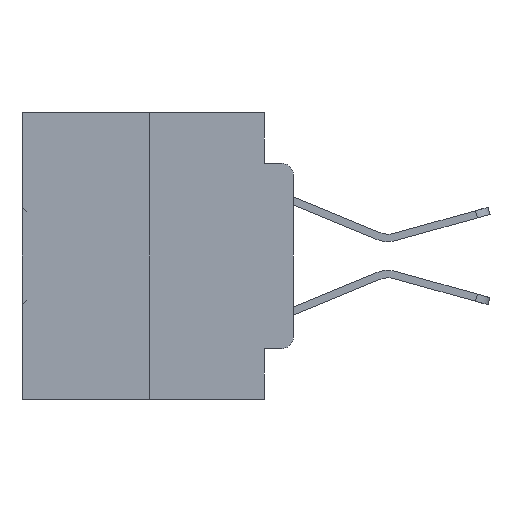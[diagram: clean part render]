
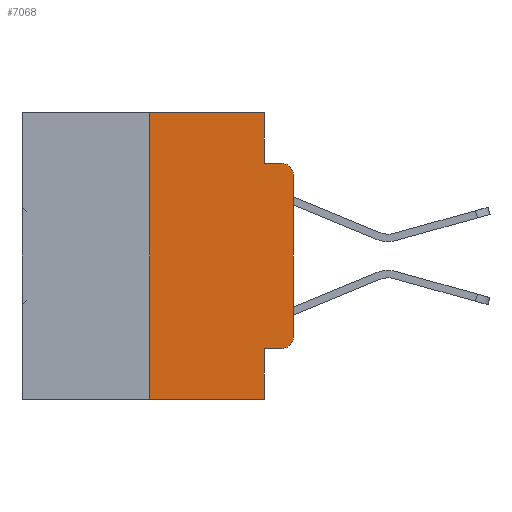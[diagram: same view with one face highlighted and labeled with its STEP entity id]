
A CAD part, left-side view. The second image highlights one B-rep face of the part: STEP entity #7068.
In plain terms, the highlighted planar face has unit normal (-1, 0, 0).
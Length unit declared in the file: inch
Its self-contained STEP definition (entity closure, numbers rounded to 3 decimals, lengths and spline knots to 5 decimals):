
#112 = AXIS2_PLACEMENT_3D ( 'NONE', #9538, #2416, #32517 ) ;
#636 = DIRECTION ( 'NONE',  ( 0., -1., 0. ) ) ;
#711 = LINE ( 'NONE', #2052, #6898 ) ;
#932 = EDGE_LOOP ( 'NONE', ( #11861, #26290, #3671, #23838, #28894, #10407, #30851, #18603, #33678, #1283 ) ) ;
#1232 = LINE ( 'NONE', #3063, #8233 ) ;
#1283 = ORIENTED_EDGE ( 'NONE', *, *, #22649, .T. ) ;
#1647 = EDGE_CURVE ( 'NONE', #32151, #18116, #25180, .T. ) ;
#2052 = CARTESIAN_POINT ( 'NONE',  ( 0., 0.051, -0.4115 ) ) ;
#2175 = CARTESIAN_POINT ( 'NONE',  ( 0., 0., -0.3915 ) ) ;
#2416 = DIRECTION ( 'NONE',  ( 1., 0., 0. ) ) ;
#2789 = CARTESIAN_POINT ( 'NONE',  ( 0., 0.25, 0. ) ) ;
#2957 = CARTESIAN_POINT ( 'NONE',  ( 0., 0., 0. ) ) ;
#3063 = CARTESIAN_POINT ( 'NONE',  ( 0., 0.473, -0.5 ) ) ;
#3671 = ORIENTED_EDGE ( 'NONE', *, *, #6938, .F. ) ;
#3848 = EDGE_CURVE ( 'NONE', #8565, #4124, #26634, .T. ) ;
#3994 = VECTOR ( 'NONE', #31921, 39.37008 ) ;
#4005 = DIRECTION ( 'NONE',  ( 0., -1., 0. ) ) ;
#4124 = VERTEX_POINT ( 'NONE', #25861 ) ;
#4366 = EDGE_CURVE ( 'NONE', #9335, #27216, #25786, .T. ) ;
#5711 = DIRECTION ( 'NONE',  ( 0., -1., 0. ) ) ;
#6165 = CARTESIAN_POINT ( 'NONE',  ( 0., 0.02, -0.3915 ) ) ;
#6453 = CARTESIAN_POINT ( 'NONE',  ( 0., 0.25, -0.5 ) ) ;
#6898 = VECTOR ( 'NONE', #25850, 39.37008 ) ;
#6938 = EDGE_CURVE ( 'NONE', #21971, #18116, #22392, .T. ) ;
#7068 = ADVANCED_FACE ( 'NONE', ( #32167 ), #7983, .F. ) ;
#7983 = PLANE ( 'NONE',  #112 ) ;
#8233 = VECTOR ( 'NONE', #5711, 39.37008 ) ;
#8385 = VECTOR ( 'NONE', #636, 39.37008 ) ;
#8565 = VERTEX_POINT ( 'NONE', #31031 ) ;
#8808 = DIRECTION ( 'NONE',  ( 0., 0., -1. ) ) ;
#8977 = LINE ( 'NONE', #2789, #29104 ) ;
#9335 = VERTEX_POINT ( 'NONE', #27362 ) ;
#9413 = CARTESIAN_POINT ( 'NONE',  ( 0., 0.051, -0.0885 ) ) ;
#9538 = CARTESIAN_POINT ( 'NONE',  ( 0., 0.473, 0. ) ) ;
#10407 = ORIENTED_EDGE ( 'NONE', *, *, #14935, .F. ) ;
#10788 = VERTEX_POINT ( 'NONE', #2175 ) ;
#11162 = CARTESIAN_POINT ( 'NONE',  ( 0., 0.051, 0. ) ) ;
#11749 = VECTOR ( 'NONE', #21383, 39.37008 ) ;
#11861 = ORIENTED_EDGE ( 'NONE', *, *, #28048, .T. ) ;
#14935 = EDGE_CURVE ( 'NONE', #27638, #8565, #8977, .T. ) ;
#15926 = DIRECTION ( 'NONE',  ( 0., 0., 1. ) ) ;
#16638 = CARTESIAN_POINT ( 'NONE',  ( 0., 0., -0.1085 ) ) ;
#16704 = EDGE_CURVE ( 'NONE', #4124, #21971, #18812, .T. ) ;
#18048 = VERTEX_POINT ( 'NONE', #24395 ) ;
#18116 = VERTEX_POINT ( 'NONE', #32456 ) ;
#18274 = CARTESIAN_POINT ( 'NONE',  ( 0., 0.051, 0. ) ) ;
#18603 = ORIENTED_EDGE ( 'NONE', *, *, #4366, .F. ) ;
#18766 = LINE ( 'NONE', #2957, #11749 ) ;
#18812 = LINE ( 'NONE', #18274, #32707 ) ;
#18856 = VECTOR ( 'NONE', #4005, 39.37008 ) ;
#19118 = CARTESIAN_POINT ( 'NONE',  ( 0., 0.051, -0.5 ) ) ;
#21383 = DIRECTION ( 'NONE',  ( 0., 0., 1. ) ) ;
#21971 = VERTEX_POINT ( 'NONE', #29742 ) ;
#22392 = LINE ( 'NONE', #9413, #8385 ) ;
#22649 = EDGE_CURVE ( 'NONE', #18048, #10788, #22736, .T. ) ;
#22736 = CIRCLE ( 'NONE', #30248, 0.02 ) ;
#23838 = ORIENTED_EDGE ( 'NONE', *, *, #16704, .F. ) ;
#24395 = CARTESIAN_POINT ( 'NONE',  ( 0., 0.02, -0.4115 ) ) ;
#24398 = EDGE_CURVE ( 'NONE', #27638, #27216, #1232, .T. ) ;
#24581 = DIRECTION ( 'NONE',  ( -1., 0., 0. ) ) ;
#25180 = CIRCLE ( 'NONE', #30174, 0.02 ) ;
#25786 = LINE ( 'NONE', #11162, #3994 ) ;
#25850 = DIRECTION ( 'NONE',  ( 0., -1., 0. ) ) ;
#25861 = CARTESIAN_POINT ( 'NONE',  ( 0., 0.051, 0. ) ) ;
#25908 = CARTESIAN_POINT ( 'NONE',  ( 0., 0.02, -0.1085 ) ) ;
#25974 = DIRECTION ( 'NONE',  ( -1., 0., 0. ) ) ;
#26144 = DIRECTION ( 'NONE',  ( 0., 0., -1. ) ) ;
#26290 = ORIENTED_EDGE ( 'NONE', *, *, #1647, .T. ) ;
#26634 = LINE ( 'NONE', #28129, #18856 ) ;
#27216 = VERTEX_POINT ( 'NONE', #19118 ) ;
#27362 = CARTESIAN_POINT ( 'NONE',  ( 0., 0.051, -0.4115 ) ) ;
#27638 = VERTEX_POINT ( 'NONE', #6453 ) ;
#28048 = EDGE_CURVE ( 'NONE', #10788, #32151, #18766, .T. ) ;
#28129 = CARTESIAN_POINT ( 'NONE',  ( 0., 0.473, 0. ) ) ;
#28673 = DIRECTION ( 'NONE',  ( 0., 0., -1. ) ) ;
#28894 = ORIENTED_EDGE ( 'NONE', *, *, #3848, .F. ) ;
#29104 = VECTOR ( 'NONE', #15926, 39.37008 ) ;
#29742 = CARTESIAN_POINT ( 'NONE',  ( 0., 0.051, -0.0885 ) ) ;
#30174 = AXIS2_PLACEMENT_3D ( 'NONE', #25908, #25974, #26144 ) ;
#30248 = AXIS2_PLACEMENT_3D ( 'NONE', #6165, #24581, #8808 ) ;
#30851 = ORIENTED_EDGE ( 'NONE', *, *, #24398, .T. ) ;
#31031 = CARTESIAN_POINT ( 'NONE',  ( 0., 0.25, 0. ) ) ;
#31921 = DIRECTION ( 'NONE',  ( 0., 0., -1. ) ) ;
#32151 = VERTEX_POINT ( 'NONE', #16638 ) ;
#32167 = FACE_OUTER_BOUND ( 'NONE', #932, .T. ) ;
#32456 = CARTESIAN_POINT ( 'NONE',  ( 0., 0.02, -0.0885 ) ) ;
#32517 = DIRECTION ( 'NONE',  ( 0., 0., -1. ) ) ;
#32707 = VECTOR ( 'NONE', #28673, 39.37008 ) ;
#33118 = EDGE_CURVE ( 'NONE', #9335, #18048, #711, .T. ) ;
#33678 = ORIENTED_EDGE ( 'NONE', *, *, #33118, .T. ) ;
